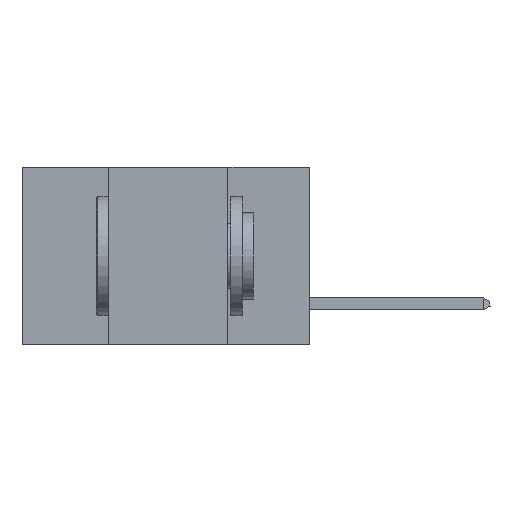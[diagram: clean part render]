
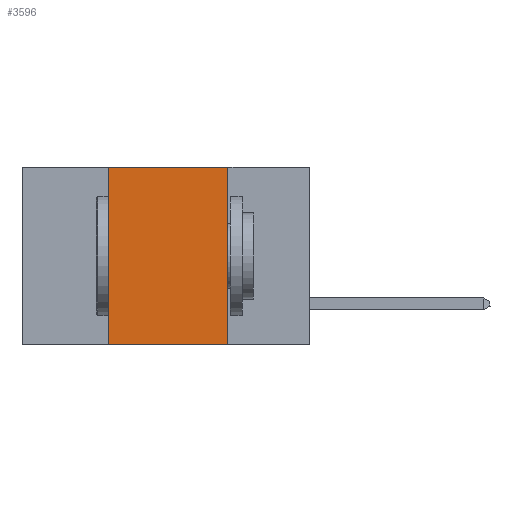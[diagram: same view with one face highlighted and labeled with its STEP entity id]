
A CAD part, left-side view. The second image highlights one B-rep face of the part: STEP entity #3596.
In plain terms, the highlighted planar face has unit normal (-1, 0, 0).
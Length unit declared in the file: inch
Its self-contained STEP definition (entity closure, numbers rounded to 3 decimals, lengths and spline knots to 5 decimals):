
#446 = VERTEX_POINT ( 'NONE', #2915 ) ;
#740 = EDGE_LOOP ( 'NONE', ( #4997, #14086, #14159, #7280 ) ) ;
#756 = CARTESIAN_POINT ( 'NONE',  ( 0., 0.17, -0.37 ) ) ;
#1323 = LINE ( 'NONE', #20055, #18318 ) ;
#1584 = DIRECTION ( 'NONE',  ( 0., 0., -1. ) ) ;
#2090 = DIRECTION ( 'NONE',  ( 0., -1., 0. ) ) ;
#2853 = LINE ( 'NONE', #9762, #4392 ) ;
#2915 = CARTESIAN_POINT ( 'NONE',  ( 0., 0.17, 0. ) ) ;
#3287 = AXIS2_PLACEMENT_3D ( 'NONE', #13285, #14889, #1584 ) ;
#3596 = ADVANCED_FACE ( 'NONE', ( #8141 ), #4942, .F. ) ;
#4336 = CARTESIAN_POINT ( 'NONE',  ( 0., 0.42, 0. ) ) ;
#4392 = VECTOR ( 'NONE', #19498, 39.37008 ) ;
#4485 = DIRECTION ( 'NONE',  ( 0., 0., 1. ) ) ;
#4649 = EDGE_CURVE ( 'NONE', #19857, #446, #1323, .T. ) ;
#4942 = PLANE ( 'NONE',  #3287 ) ;
#4997 = ORIENTED_EDGE ( 'NONE', *, *, #19792, .F. ) ;
#5395 = DIRECTION ( 'NONE',  ( 0., -1., 0. ) ) ;
#7280 = ORIENTED_EDGE ( 'NONE', *, *, #17734, .T. ) ;
#8141 = FACE_OUTER_BOUND ( 'NONE', #740, .T. ) ;
#9762 = CARTESIAN_POINT ( 'NONE',  ( 0., 0.17, 0. ) ) ;
#11990 = EDGE_CURVE ( 'NONE', #16057, #19857, #16857, .T. ) ;
#12261 = CARTESIAN_POINT ( 'NONE',  ( 0., 0.42, -0.37 ) ) ;
#13285 = CARTESIAN_POINT ( 'NONE',  ( 0., 0.6, 0. ) ) ;
#13613 = CARTESIAN_POINT ( 'NONE',  ( 0., 0.6, -0.37 ) ) ;
#14086 = ORIENTED_EDGE ( 'NONE', *, *, #4649, .F. ) ;
#14159 = ORIENTED_EDGE ( 'NONE', *, *, #11990, .F. ) ;
#14783 = VERTEX_POINT ( 'NONE', #756 ) ;
#14889 = DIRECTION ( 'NONE',  ( 1., 0., 0. ) ) ;
#16057 = VERTEX_POINT ( 'NONE', #12261 ) ;
#16857 = LINE ( 'NONE', #4336, #17621 ) ;
#16866 = VECTOR ( 'NONE', #5395, 39.37008 ) ;
#17621 = VECTOR ( 'NONE', #4485, 39.37008 ) ;
#17734 = EDGE_CURVE ( 'NONE', #16057, #14783, #21205, .T. ) ;
#18318 = VECTOR ( 'NONE', #2090, 39.37008 ) ;
#19498 = DIRECTION ( 'NONE',  ( 0., 0., -1. ) ) ;
#19792 = EDGE_CURVE ( 'NONE', #446, #14783, #2853, .T. ) ;
#19857 = VERTEX_POINT ( 'NONE', #21124 ) ;
#20055 = CARTESIAN_POINT ( 'NONE',  ( 0., 0.6, 0. ) ) ;
#21124 = CARTESIAN_POINT ( 'NONE',  ( 0., 0.42, 0. ) ) ;
#21205 = LINE ( 'NONE', #13613, #16866 ) ;
